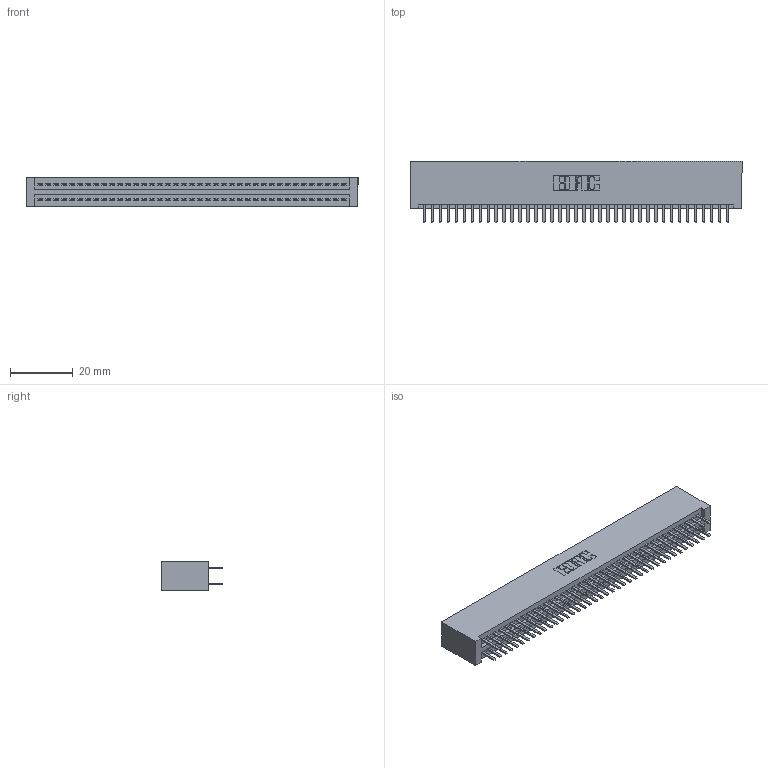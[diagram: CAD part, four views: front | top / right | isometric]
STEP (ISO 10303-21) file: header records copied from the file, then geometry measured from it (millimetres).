
FILE_DESCRIPTION (( 'STEP AP203' ), '1' );
FILE_NAME ('345-078-520-201.STEP', '2018-10-02T19:14:07', ( '' ), ( '' ), 'SwSTEP 2.0', 'SolidWorks 2016', '' );
FILE_SCHEMA (( 'CONFIG_CONTROL_DESIGN' ));
Length unit declared in the file: inch
Products named in the file (3): 345 Part_No Mounting Lugs; 345-292-001_345-293-120; 345-078-520-201
Assembly tree (79 placements, depth 2):
  345-078-520-201
    345 Part_No Mounting Lugs
    345-292-001_345-293-120  x78
Bounding box: 105.66 x 19.68 x 9.4 mm (x, y, z)
Volume: 10818.1 mm3; surface area: 16163.2 mm2
Topology: 79 solids, 79 shells, 4330 faces, 12563 edges, 8166 vertices
Faces by surface type: plane 2806, cylinder 1524
Entity records: 30841 total; most frequent: CARTESIAN_POINT 5184, ORIENTED_EDGE 5106, DIRECTION 4557, EDGE_CURVE 2553, LINE 2269, VECTOR 2269, VERTEX_POINT 1698, AXIS2_PLACEMENT_3D 1144
